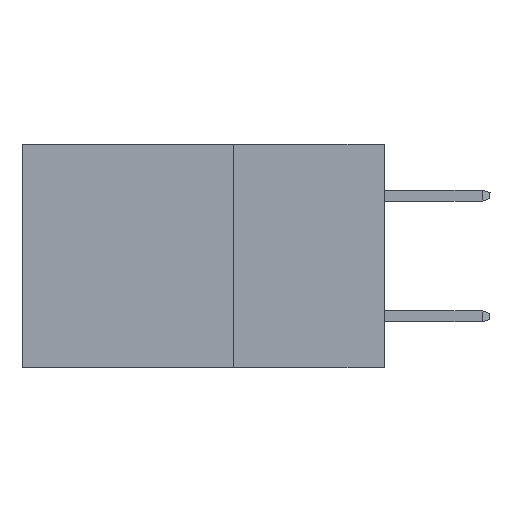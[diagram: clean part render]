
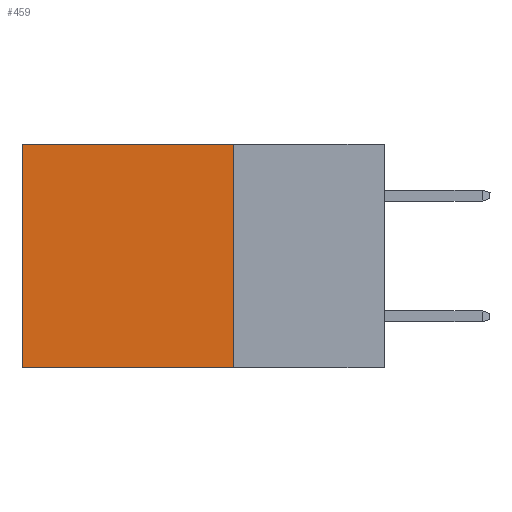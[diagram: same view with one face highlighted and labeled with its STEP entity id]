
A CAD part, left-side view. The second image highlights one B-rep face of the part: STEP entity #459.
In plain terms, the highlighted planar face has unit normal (-1, 0, 0).
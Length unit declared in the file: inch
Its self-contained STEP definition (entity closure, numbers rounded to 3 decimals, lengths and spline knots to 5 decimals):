
#459 = ADVANCED_FACE ( 'NONE', ( #12766 ), #8009, .F. ) ;
#545 = VECTOR ( 'NONE', #16089, 39.37008 ) ;
#2244 = VERTEX_POINT ( 'NONE', #11776 ) ;
#2249 = DIRECTION ( 'NONE',  ( 0., 0., -1. ) ) ;
#2644 = VERTEX_POINT ( 'NONE', #10060 ) ;
#2807 = AXIS2_PLACEMENT_3D ( 'NONE', #16660, #7970, #6864 ) ;
#3062 = ORIENTED_EDGE ( 'NONE', *, *, #16380, .T. ) ;
#3780 = CARTESIAN_POINT ( 'NONE',  ( 0.298, 0.6, 0. ) ) ;
#4148 = LINE ( 'NONE', #5486, #545 ) ;
#4295 = CARTESIAN_POINT ( 'NONE',  ( 0.298, 0.25, 0. ) ) ;
#5446 = CARTESIAN_POINT ( 'NONE',  ( 0.298, 0.25, -0.37 ) ) ;
#5486 = CARTESIAN_POINT ( 'NONE',  ( 0.298, 0.25, 0. ) ) ;
#5822 = DIRECTION ( 'NONE',  ( 0., 0., -1. ) ) ;
#5942 = EDGE_LOOP ( 'NONE', ( #3062, #8991, #11472, #13120 ) ) ;
#6066 = VERTEX_POINT ( 'NONE', #6819 ) ;
#6787 = EDGE_CURVE ( 'NONE', #6066, #2244, #10398, .T. ) ;
#6819 = CARTESIAN_POINT ( 'NONE',  ( 0.298, 0.25, -0.37 ) ) ;
#6864 = DIRECTION ( 'NONE',  ( 0., 0., -1. ) ) ;
#7970 = DIRECTION ( 'NONE',  ( 1., 0., 0. ) ) ;
#8009 = PLANE ( 'NONE',  #2807 ) ;
#8991 = ORIENTED_EDGE ( 'NONE', *, *, #6787, .F. ) ;
#9081 = CARTESIAN_POINT ( 'NONE',  ( 0.298, 0.25, 0. ) ) ;
#10060 = CARTESIAN_POINT ( 'NONE',  ( 0.298, 0.6, 0. ) ) ;
#10123 = EDGE_CURVE ( 'NONE', #12357, #6066, #10579, .T. ) ;
#10398 = LINE ( 'NONE', #5446, #18427 ) ;
#10579 = LINE ( 'NONE', #4295, #14195 ) ;
#10659 = EDGE_CURVE ( 'NONE', #12357, #2644, #4148, .T. ) ;
#11472 = ORIENTED_EDGE ( 'NONE', *, *, #10123, .F. ) ;
#11776 = CARTESIAN_POINT ( 'NONE',  ( 0.298, 0.6, -0.37 ) ) ;
#12357 = VERTEX_POINT ( 'NONE', #9081 ) ;
#12766 = FACE_OUTER_BOUND ( 'NONE', #5942, .T. ) ;
#13120 = ORIENTED_EDGE ( 'NONE', *, *, #10659, .T. ) ;
#13278 = VECTOR ( 'NONE', #2249, 39.37008 ) ;
#14195 = VECTOR ( 'NONE', #5822, 39.37008 ) ;
#16033 = DIRECTION ( 'NONE',  ( 0., 1., 0. ) ) ;
#16089 = DIRECTION ( 'NONE',  ( 0., 1., 0. ) ) ;
#16380 = EDGE_CURVE ( 'NONE', #2644, #2244, #17295, .T. ) ;
#16660 = CARTESIAN_POINT ( 'NONE',  ( 0.298, 0.25, 0. ) ) ;
#17295 = LINE ( 'NONE', #3780, #13278 ) ;
#18427 = VECTOR ( 'NONE', #16033, 39.37008 ) ;
